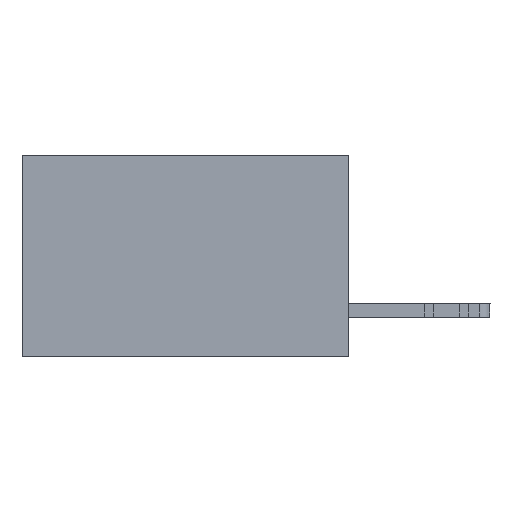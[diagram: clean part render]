
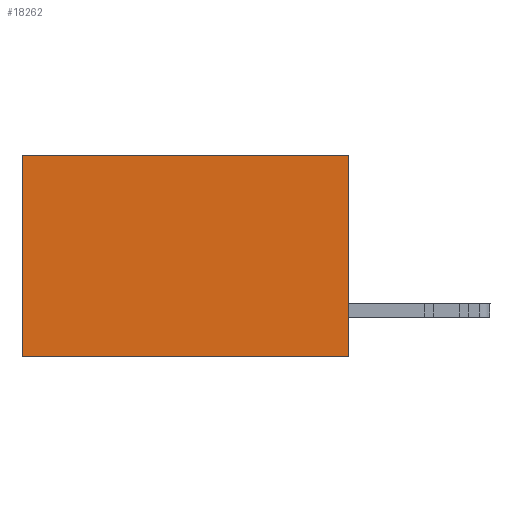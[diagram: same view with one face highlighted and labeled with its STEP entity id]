
A CAD part, left-side view. The second image highlights one B-rep face of the part: STEP entity #18262.
In plain terms, the highlighted planar face has unit normal (-1, 0, 0).
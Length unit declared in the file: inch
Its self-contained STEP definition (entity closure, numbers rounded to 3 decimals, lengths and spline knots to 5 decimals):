
#336 = DIRECTION ( 'NONE',  ( 0., 0., -1. ) ) ;
#604 = LINE ( 'NONE', #2144, #17666 ) ;
#1790 = CARTESIAN_POINT ( 'NONE',  ( 0.2615, 0., 0. ) ) ;
#2116 = DIRECTION ( 'NONE',  ( 1., 0., 0. ) ) ;
#2144 = CARTESIAN_POINT ( 'NONE',  ( 0.2615, 0., -0.37 ) ) ;
#2992 = VERTEX_POINT ( 'NONE', #12331 ) ;
#3201 = EDGE_CURVE ( 'NONE', #13927, #18316, #604, .T. ) ;
#4857 = VECTOR ( 'NONE', #12812, 39.37008 ) ;
#5232 = DIRECTION ( 'NONE',  ( 0., 1., 0. ) ) ;
#5263 = EDGE_LOOP ( 'NONE', ( #23086, #12591, #5783, #16310 ) ) ;
#5783 = ORIENTED_EDGE ( 'NONE', *, *, #6195, .F. ) ;
#6195 = EDGE_CURVE ( 'NONE', #14990, #13927, #16608, .T. ) ;
#6298 = CARTESIAN_POINT ( 'NONE',  ( 0.2615, 0., -0.37 ) ) ;
#8137 = AXIS2_PLACEMENT_3D ( 'NONE', #17583, #2116, #336 ) ;
#8850 = VECTOR ( 'NONE', #5232, 39.37008 ) ;
#9121 = CARTESIAN_POINT ( 'NONE',  ( 0.2615, 0., 0. ) ) ;
#10071 = CARTESIAN_POINT ( 'NONE',  ( 0.2615, 0.6, -0.37 ) ) ;
#10132 = FACE_OUTER_BOUND ( 'NONE', #5263, .T. ) ;
#12331 = CARTESIAN_POINT ( 'NONE',  ( 0.2615, 0.6, 0. ) ) ;
#12591 = ORIENTED_EDGE ( 'NONE', *, *, #3201, .F. ) ;
#12812 = DIRECTION ( 'NONE',  ( 0., 0., -1. ) ) ;
#13927 = VERTEX_POINT ( 'NONE', #6298 ) ;
#14915 = LINE ( 'NONE', #9121, #8850 ) ;
#14990 = VERTEX_POINT ( 'NONE', #1790 ) ;
#16310 = ORIENTED_EDGE ( 'NONE', *, *, #24583, .T. ) ;
#16608 = LINE ( 'NONE', #22765, #4857 ) ;
#17583 = CARTESIAN_POINT ( 'NONE',  ( 0.2615, 0., -0.37 ) ) ;
#17666 = VECTOR ( 'NONE', #23145, 39.37008 ) ;
#17765 = LINE ( 'NONE', #10071, #24081 ) ;
#18262 = ADVANCED_FACE ( 'NONE', ( #10132 ), #21232, .F. ) ;
#18316 = VERTEX_POINT ( 'NONE', #23856 ) ;
#19771 = DIRECTION ( 'NONE',  ( 0., 0., -1. ) ) ;
#21232 = PLANE ( 'NONE',  #8137 ) ;
#22256 = EDGE_CURVE ( 'NONE', #2992, #18316, #17765, .T. ) ;
#22765 = CARTESIAN_POINT ( 'NONE',  ( 0.2615, 0., -0.37 ) ) ;
#23086 = ORIENTED_EDGE ( 'NONE', *, *, #22256, .T. ) ;
#23145 = DIRECTION ( 'NONE',  ( 0., 1., 0. ) ) ;
#23856 = CARTESIAN_POINT ( 'NONE',  ( 0.2615, 0.6, -0.37 ) ) ;
#24081 = VECTOR ( 'NONE', #19771, 39.37008 ) ;
#24583 = EDGE_CURVE ( 'NONE', #14990, #2992, #14915, .T. ) ;
